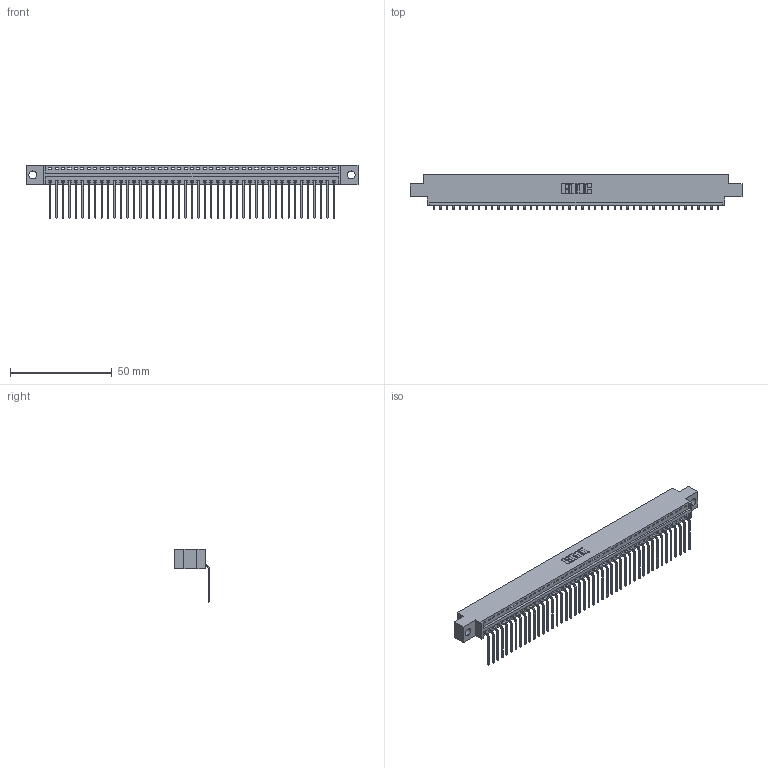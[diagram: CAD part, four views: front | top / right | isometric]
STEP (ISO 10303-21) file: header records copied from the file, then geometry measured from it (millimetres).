
FILE_DESCRIPTION (( 'STEP AP203' ), '1' );
FILE_NAME ('396-045-559-604.STEP', '2018-09-07T06:59:52', ( '' ), ( '' ), 'SwSTEP 2.0', 'SolidWorks 2016', '' );
FILE_SCHEMA (( 'CONFIG_CONTROL_DESIGN' ));
Length unit declared in the file: inch
Products named in the file (3): 346 Part_0.170 Offset - 0.156 Dia-TH; 345-292-001_558 559 Tail - 1; 396-045-559-604
Assembly tree (46 placements, depth 2):
  396-045-559-604
    346 Part_0.170 Offset - 0.156 Dia-TH
    345-292-001_558 559 Tail - 1  x45
Bounding box: 163.45 x 17.08 x 26.16 mm (x, y, z)
Volume: 15573.8 mm3; surface area: 20357.4 mm2
Topology: 46 solids, 46 shells, 2826 faces, 8531 edges, 5626 vertices
Faces by surface type: plane 1970, cylinder 856
Entity records: 27743 total; most frequent: CARTESIAN_POINT 4763, ORIENTED_EDGE 4742, DIRECTION 4197, EDGE_CURVE 2371, LINE 2059, VECTOR 2059, VERTEX_POINT 1578, AXIS2_PLACEMENT_3D 1069
